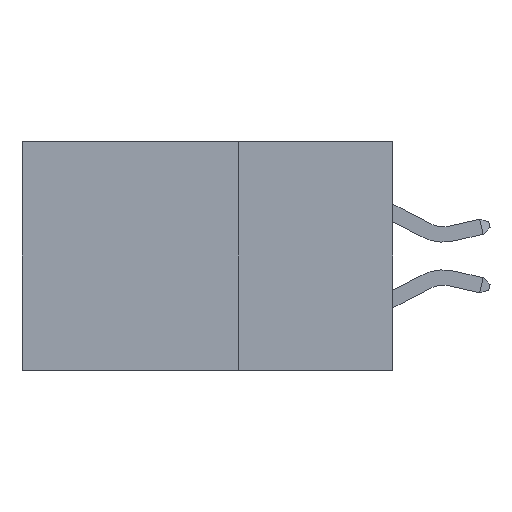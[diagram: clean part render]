
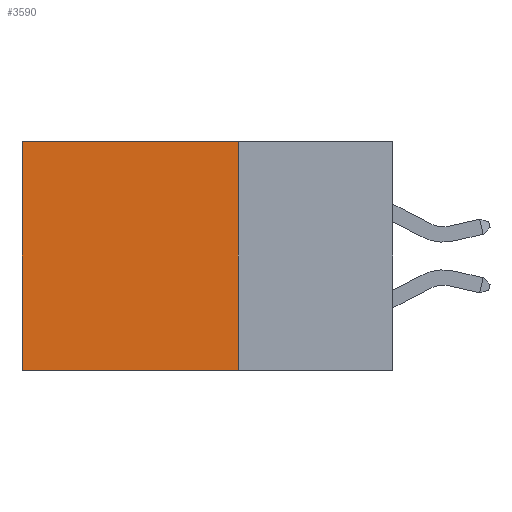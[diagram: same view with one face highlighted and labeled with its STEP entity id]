
A CAD part, left-side view. The second image highlights one B-rep face of the part: STEP entity #3590.
In plain terms, the highlighted planar face has unit normal (-1, 0, 0).
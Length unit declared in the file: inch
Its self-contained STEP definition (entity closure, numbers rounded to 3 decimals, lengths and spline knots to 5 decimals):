
#138 = VECTOR ( 'NONE', #7371, 39.37008 ) ;
#222 = ORIENTED_EDGE ( 'NONE', *, *, #9969, .F. ) ;
#1769 = ORIENTED_EDGE ( 'NONE', *, *, #7252, .F. ) ;
#2246 = DIRECTION ( 'NONE',  ( 0., 0., -1. ) ) ;
#3590 = ADVANCED_FACE ( 'NONE', ( #7167 ), #16759, .F. ) ;
#3944 = VECTOR ( 'NONE', #11980, 39.37008 ) ;
#4149 = DIRECTION ( 'NONE',  ( 0., 0., -1. ) ) ;
#6212 = EDGE_CURVE ( 'NONE', #10802, #7893, #9670, .T. ) ;
#7075 = ORIENTED_EDGE ( 'NONE', *, *, #6212, .T. ) ;
#7167 = FACE_OUTER_BOUND ( 'NONE', #13529, .T. ) ;
#7252 = EDGE_CURVE ( 'NONE', #14291, #7893, #8634, .T. ) ;
#7371 = DIRECTION ( 'NONE',  ( 0., 0., -1. ) ) ;
#7431 = CARTESIAN_POINT ( 'NONE',  ( 0.2875, 0.25, 0. ) ) ;
#7468 = CARTESIAN_POINT ( 'NONE',  ( 0.2875, 0.6, 0. ) ) ;
#7676 = DIRECTION ( 'NONE',  ( 1., 0., 0. ) ) ;
#7893 = VERTEX_POINT ( 'NONE', #13493 ) ;
#8297 = AXIS2_PLACEMENT_3D ( 'NONE', #14279, #7676, #4149 ) ;
#8634 = LINE ( 'NONE', #14497, #3944 ) ;
#9083 = CARTESIAN_POINT ( 'NONE',  ( 0.2875, 0.25, 0. ) ) ;
#9670 = LINE ( 'NONE', #7468, #138 ) ;
#9969 = EDGE_CURVE ( 'NONE', #13464, #14291, #10452, .T. ) ;
#10452 = LINE ( 'NONE', #7431, #14534 ) ;
#10802 = VERTEX_POINT ( 'NONE', #13147 ) ;
#11110 = CARTESIAN_POINT ( 'NONE',  ( 0.2875, 0.25, 0. ) ) ;
#11564 = CARTESIAN_POINT ( 'NONE',  ( 0.2875, 0.25, -0.37 ) ) ;
#11980 = DIRECTION ( 'NONE',  ( 0., 1., 0. ) ) ;
#11993 = EDGE_CURVE ( 'NONE', #13464, #10802, #12650, .T. ) ;
#12650 = LINE ( 'NONE', #9083, #15295 ) ;
#12972 = DIRECTION ( 'NONE',  ( 0., 1., 0. ) ) ;
#13147 = CARTESIAN_POINT ( 'NONE',  ( 0.2875, 0.6, 0. ) ) ;
#13464 = VERTEX_POINT ( 'NONE', #11110 ) ;
#13493 = CARTESIAN_POINT ( 'NONE',  ( 0.2875, 0.6, -0.37 ) ) ;
#13529 = EDGE_LOOP ( 'NONE', ( #7075, #1769, #222, #13885 ) ) ;
#13885 = ORIENTED_EDGE ( 'NONE', *, *, #11993, .T. ) ;
#14279 = CARTESIAN_POINT ( 'NONE',  ( 0.2875, 0.25, 0. ) ) ;
#14291 = VERTEX_POINT ( 'NONE', #11564 ) ;
#14497 = CARTESIAN_POINT ( 'NONE',  ( 0.2875, 0.25, -0.37 ) ) ;
#14534 = VECTOR ( 'NONE', #2246, 39.37008 ) ;
#15295 = VECTOR ( 'NONE', #12972, 39.37008 ) ;
#16759 = PLANE ( 'NONE',  #8297 ) ;
